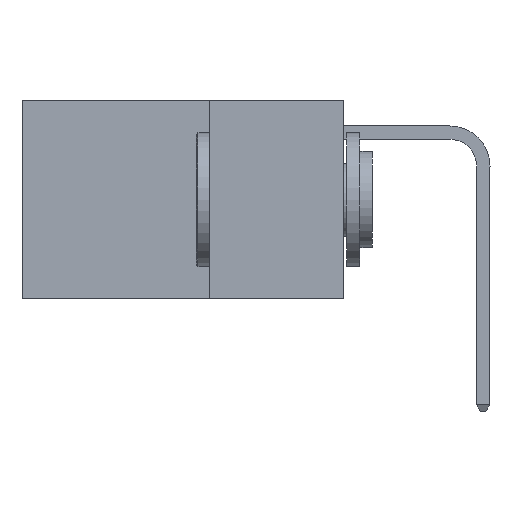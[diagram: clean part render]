
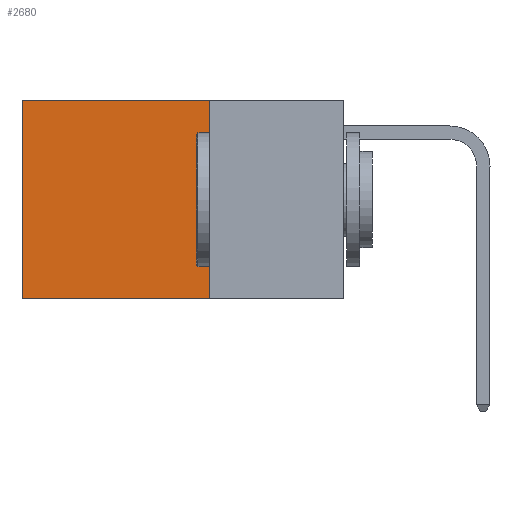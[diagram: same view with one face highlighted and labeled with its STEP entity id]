
A CAD part, left-side view. The second image highlights one B-rep face of the part: STEP entity #2680.
In plain terms, the highlighted planar face has unit normal (-1, 0, 0).
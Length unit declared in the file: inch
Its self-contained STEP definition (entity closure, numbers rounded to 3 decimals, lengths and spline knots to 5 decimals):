
#65 = VECTOR ( 'NONE', #1985, 39.37008 ) ;
#470 = DIRECTION ( 'NONE',  ( 0., 1., 0. ) ) ;
#1727 = CARTESIAN_POINT ( 'NONE',  ( 0.2625, 0.25, 0. ) ) ;
#1985 = DIRECTION ( 'NONE',  ( 0., 0., -1. ) ) ;
#2680 = ADVANCED_FACE ( 'NONE', ( #6043 ), #4514, .F. ) ;
#2983 = EDGE_LOOP ( 'NONE', ( #12348, #12644, #6265, #4386 ) ) ;
#3148 = DIRECTION ( 'NONE',  ( 0., 0., -1. ) ) ;
#3649 = LINE ( 'NONE', #16724, #14075 ) ;
#3796 = LINE ( 'NONE', #15533, #65 ) ;
#4161 = LINE ( 'NONE', #11799, #14547 ) ;
#4386 = ORIENTED_EDGE ( 'NONE', *, *, #14393, .T. ) ;
#4514 = PLANE ( 'NONE',  #16534 ) ;
#5482 = EDGE_CURVE ( 'NONE', #11956, #10499, #12757, .T. ) ;
#5599 = EDGE_CURVE ( 'NONE', #9655, #7921, #3796, .T. ) ;
#5892 = DIRECTION ( 'NONE',  ( 0., 0., -1. ) ) ;
#6043 = FACE_OUTER_BOUND ( 'NONE', #2983, .T. ) ;
#6265 = ORIENTED_EDGE ( 'NONE', *, *, #5599, .F. ) ;
#7921 = VERTEX_POINT ( 'NONE', #8461 ) ;
#8461 = CARTESIAN_POINT ( 'NONE',  ( 0.2625, 0.25, -0.37 ) ) ;
#8548 = CARTESIAN_POINT ( 'NONE',  ( 0.2625, 0.6, -0.37 ) ) ;
#9187 = VECTOR ( 'NONE', #3148, 39.37008 ) ;
#9655 = VERTEX_POINT ( 'NONE', #17218 ) ;
#10499 = VERTEX_POINT ( 'NONE', #8548 ) ;
#11799 = CARTESIAN_POINT ( 'NONE',  ( 0.2625, 0.25, -0.37 ) ) ;
#11956 = VERTEX_POINT ( 'NONE', #15582 ) ;
#12348 = ORIENTED_EDGE ( 'NONE', *, *, #5482, .T. ) ;
#12565 = EDGE_CURVE ( 'NONE', #7921, #10499, #4161, .T. ) ;
#12644 = ORIENTED_EDGE ( 'NONE', *, *, #12565, .F. ) ;
#12757 = LINE ( 'NONE', #16610, #9187 ) ;
#14025 = DIRECTION ( 'NONE',  ( 1., 0., 0. ) ) ;
#14075 = VECTOR ( 'NONE', #470, 39.37008 ) ;
#14393 = EDGE_CURVE ( 'NONE', #9655, #11956, #3649, .T. ) ;
#14547 = VECTOR ( 'NONE', #15786, 39.37008 ) ;
#15533 = CARTESIAN_POINT ( 'NONE',  ( 0.2625, 0.25, 0. ) ) ;
#15582 = CARTESIAN_POINT ( 'NONE',  ( 0.2625, 0.6, 0. ) ) ;
#15786 = DIRECTION ( 'NONE',  ( 0., 1., 0. ) ) ;
#16534 = AXIS2_PLACEMENT_3D ( 'NONE', #1727, #14025, #5892 ) ;
#16610 = CARTESIAN_POINT ( 'NONE',  ( 0.2625, 0.6, 0. ) ) ;
#16724 = CARTESIAN_POINT ( 'NONE',  ( 0.2625, 0.25, 0. ) ) ;
#17218 = CARTESIAN_POINT ( 'NONE',  ( 0.2625, 0.25, 0. ) ) ;
